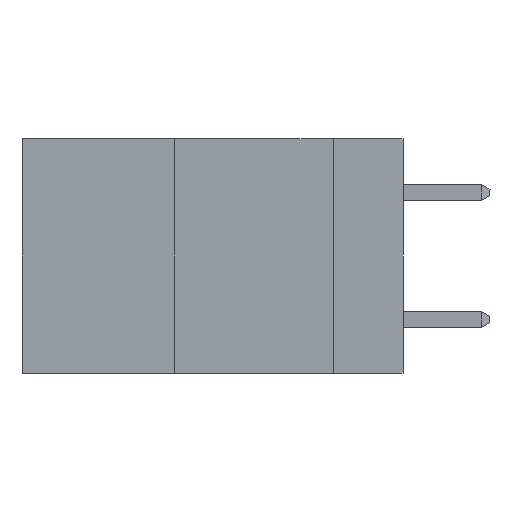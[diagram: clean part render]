
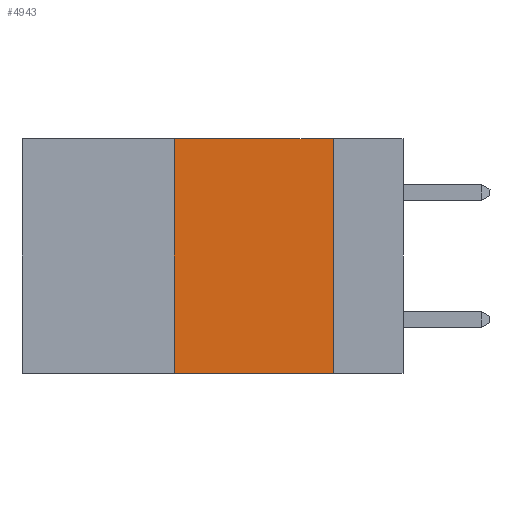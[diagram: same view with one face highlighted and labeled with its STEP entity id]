
A CAD part, left-side view. The second image highlights one B-rep face of the part: STEP entity #4943.
In plain terms, the highlighted planar face has unit normal (-1, 0, 0).
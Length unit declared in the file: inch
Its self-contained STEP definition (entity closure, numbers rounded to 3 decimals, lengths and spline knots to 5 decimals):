
#739 = ORIENTED_EDGE ( 'NONE', *, *, #2404, .T. ) ;
#1702 = CARTESIAN_POINT ( 'NONE',  ( 0., 0.36, -0.37 ) ) ;
#2019 = DIRECTION ( 'NONE',  ( 1., 0., 0. ) ) ;
#2300 = VERTEX_POINT ( 'NONE', #10157 ) ;
#2404 = EDGE_CURVE ( 'NONE', #9449, #9419, #3046, .T. ) ;
#2946 = VECTOR ( 'NONE', #13769, 39.37008 ) ;
#3046 = LINE ( 'NONE', #4194, #11526 ) ;
#3284 = DIRECTION ( 'NONE',  ( 0., -1., 0. ) ) ;
#3361 = PLANE ( 'NONE',  #8533 ) ;
#3503 = CARTESIAN_POINT ( 'NONE',  ( 0., 0.36, 0. ) ) ;
#3684 = CARTESIAN_POINT ( 'NONE',  ( 0., 0.11, -0.37 ) ) ;
#3828 = VERTEX_POINT ( 'NONE', #3503 ) ;
#4194 = CARTESIAN_POINT ( 'NONE',  ( 0., 0.6, -0.37 ) ) ;
#4287 = ORIENTED_EDGE ( 'NONE', *, *, #12518, .F. ) ;
#4714 = EDGE_LOOP ( 'NONE', ( #4287, #9211, #12545, #739 ) ) ;
#4791 = VECTOR ( 'NONE', #3284, 39.37008 ) ;
#4943 = ADVANCED_FACE ( 'NONE', ( #10696 ), #3361, .F. ) ;
#5340 = CARTESIAN_POINT ( 'NONE',  ( 0., 0.6, 0. ) ) ;
#5884 = DIRECTION ( 'NONE',  ( 0., 0., 1. ) ) ;
#6434 = CARTESIAN_POINT ( 'NONE',  ( 0., 0.6, 0. ) ) ;
#6568 = DIRECTION ( 'NONE',  ( 0., 0., -1. ) ) ;
#7314 = DIRECTION ( 'NONE',  ( 0., -1., 0. ) ) ;
#7685 = LINE ( 'NONE', #5340, #4791 ) ;
#8440 = LINE ( 'NONE', #12780, #2946 ) ;
#8533 = AXIS2_PLACEMENT_3D ( 'NONE', #6434, #2019, #6568 ) ;
#9211 = ORIENTED_EDGE ( 'NONE', *, *, #13632, .F. ) ;
#9419 = VERTEX_POINT ( 'NONE', #3684 ) ;
#9449 = VERTEX_POINT ( 'NONE', #1702 ) ;
#9525 = EDGE_CURVE ( 'NONE', #9449, #3828, #12506, .T. ) ;
#10157 = CARTESIAN_POINT ( 'NONE',  ( 0., 0.11, 0. ) ) ;
#10293 = CARTESIAN_POINT ( 'NONE',  ( 0., 0.36, 0. ) ) ;
#10696 = FACE_OUTER_BOUND ( 'NONE', #4714, .T. ) ;
#11526 = VECTOR ( 'NONE', #7314, 39.37008 ) ;
#11787 = VECTOR ( 'NONE', #5884, 39.37008 ) ;
#12506 = LINE ( 'NONE', #10293, #11787 ) ;
#12518 = EDGE_CURVE ( 'NONE', #2300, #9419, #8440, .T. ) ;
#12545 = ORIENTED_EDGE ( 'NONE', *, *, #9525, .F. ) ;
#12780 = CARTESIAN_POINT ( 'NONE',  ( 0., 0.11, 0. ) ) ;
#13632 = EDGE_CURVE ( 'NONE', #3828, #2300, #7685, .T. ) ;
#13769 = DIRECTION ( 'NONE',  ( 0., 0., -1. ) ) ;
